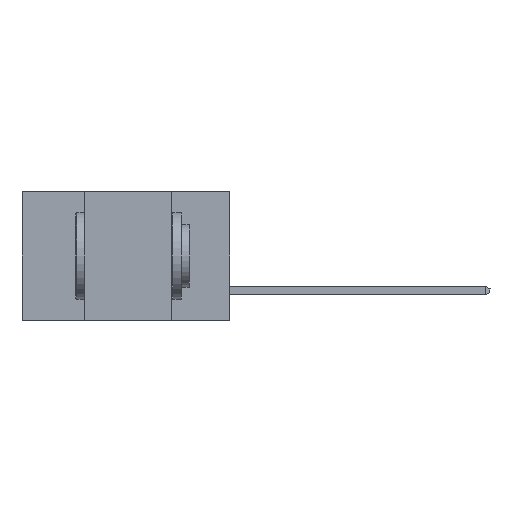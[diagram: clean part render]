
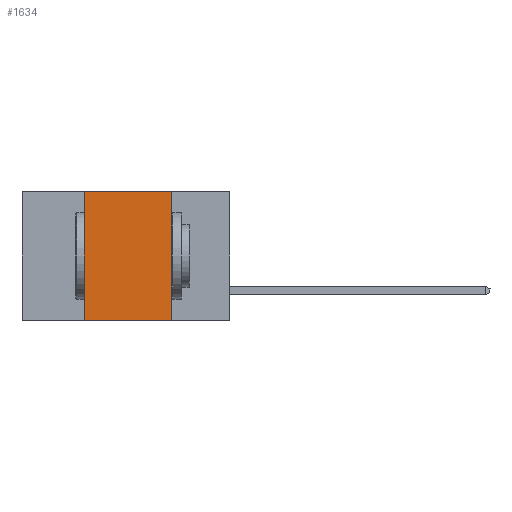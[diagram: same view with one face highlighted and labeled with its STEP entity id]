
A CAD part, left-side view. The second image highlights one B-rep face of the part: STEP entity #1634.
In plain terms, the highlighted planar face has unit normal (-1, 0, 0).
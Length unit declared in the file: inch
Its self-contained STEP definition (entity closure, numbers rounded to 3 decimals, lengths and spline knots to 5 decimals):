
#1027 = CARTESIAN_POINT ( 'NONE',  ( 0., 0.42, 0. ) ) ;
#1634 = ADVANCED_FACE ( 'NONE', ( #4540 ), #12774, .F. ) ;
#1639 = LINE ( 'NONE', #8376, #6169 ) ;
#1846 = DIRECTION ( 'NONE',  ( 0., 0., 1. ) ) ;
#2219 = LINE ( 'NONE', #6838, #12146 ) ;
#2287 = CARTESIAN_POINT ( 'NONE',  ( 0., 0.42, -0.37 ) ) ;
#3394 = VERTEX_POINT ( 'NONE', #2287 ) ;
#3561 = CARTESIAN_POINT ( 'NONE',  ( 0., 0.6, 0. ) ) ;
#4540 = FACE_OUTER_BOUND ( 'NONE', #12054, .T. ) ;
#4621 = ORIENTED_EDGE ( 'NONE', *, *, #6660, .T. ) ;
#5617 = EDGE_CURVE ( 'NONE', #13727, #12352, #1639, .T. ) ;
#5887 = ORIENTED_EDGE ( 'NONE', *, *, #9791, .F. ) ;
#6169 = VECTOR ( 'NONE', #6253, 39.37008 ) ;
#6253 = DIRECTION ( 'NONE',  ( 0., -1., 0. ) ) ;
#6660 = EDGE_CURVE ( 'NONE', #3394, #9372, #14437, .T. ) ;
#6838 = CARTESIAN_POINT ( 'NONE',  ( 0., 0.17, -0.37 ) ) ;
#6884 = AXIS2_PLACEMENT_3D ( 'NONE', #3561, #10362, #11492 ) ;
#7595 = LINE ( 'NONE', #12178, #11122 ) ;
#8376 = CARTESIAN_POINT ( 'NONE',  ( 0., 0.6, 0. ) ) ;
#8734 = CARTESIAN_POINT ( 'NONE',  ( 0., 0.17, 0. ) ) ;
#9372 = VERTEX_POINT ( 'NONE', #13760 ) ;
#9791 = EDGE_CURVE ( 'NONE', #3394, #13727, #7595, .T. ) ;
#9869 = ORIENTED_EDGE ( 'NONE', *, *, #5617, .F. ) ;
#10362 = DIRECTION ( 'NONE',  ( 1., 0., 0. ) ) ;
#11122 = VECTOR ( 'NONE', #1846, 39.37008 ) ;
#11215 = DIRECTION ( 'NONE',  ( 0., -1., 0. ) ) ;
#11435 = DIRECTION ( 'NONE',  ( 0., 0., -1. ) ) ;
#11492 = DIRECTION ( 'NONE',  ( 0., 0., -1. ) ) ;
#12054 = EDGE_LOOP ( 'NONE', ( #12702, #9869, #5887, #4621 ) ) ;
#12146 = VECTOR ( 'NONE', #11435, 39.37008 ) ;
#12178 = CARTESIAN_POINT ( 'NONE',  ( 0., 0.42, -0.37 ) ) ;
#12352 = VERTEX_POINT ( 'NONE', #8734 ) ;
#12702 = ORIENTED_EDGE ( 'NONE', *, *, #14307, .F. ) ;
#12774 = PLANE ( 'NONE',  #6884 ) ;
#13727 = VERTEX_POINT ( 'NONE', #1027 ) ;
#13760 = CARTESIAN_POINT ( 'NONE',  ( 0., 0.17, -0.37 ) ) ;
#13955 = VECTOR ( 'NONE', #11215, 39.37008 ) ;
#14307 = EDGE_CURVE ( 'NONE', #12352, #9372, #2219, .T. ) ;
#14437 = LINE ( 'NONE', #14591, #13955 ) ;
#14591 = CARTESIAN_POINT ( 'NONE',  ( 0., 0.6, -0.37 ) ) ;
